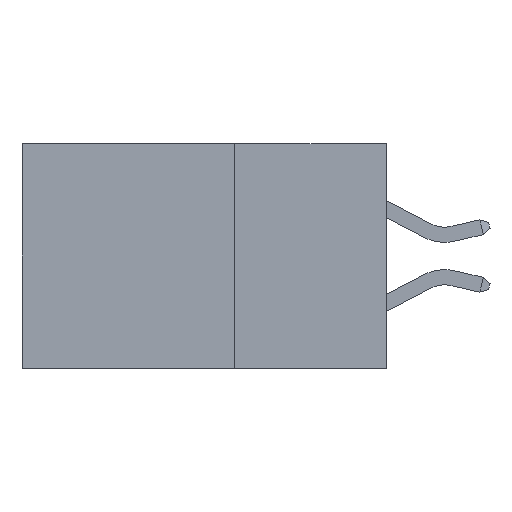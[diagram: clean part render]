
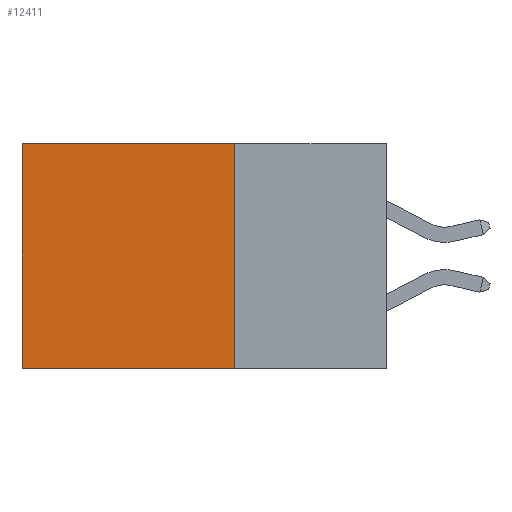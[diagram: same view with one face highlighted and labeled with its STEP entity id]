
A CAD part, left-side view. The second image highlights one B-rep face of the part: STEP entity #12411.
In plain terms, the highlighted planar face has unit normal (-1, 0, 0).
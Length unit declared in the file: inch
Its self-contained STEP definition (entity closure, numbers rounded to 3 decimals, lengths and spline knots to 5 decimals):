
#484 = CARTESIAN_POINT ( 'NONE',  ( 0.298, 0.6, 0. ) ) ;
#1757 = FACE_OUTER_BOUND ( 'NONE', #4726, .T. ) ;
#2132 = VERTEX_POINT ( 'NONE', #3837 ) ;
#2799 = VECTOR ( 'NONE', #9024, 39.37008 ) ;
#3102 = CARTESIAN_POINT ( 'NONE',  ( 0.298, 0.6, -0.37 ) ) ;
#3278 = ORIENTED_EDGE ( 'NONE', *, *, #11092, .F. ) ;
#3798 = VERTEX_POINT ( 'NONE', #9820 ) ;
#3837 = CARTESIAN_POINT ( 'NONE',  ( 0.298, 0.25, -0.37 ) ) ;
#4545 = VECTOR ( 'NONE', #10552, 39.37008 ) ;
#4726 = EDGE_LOOP ( 'NONE', ( #4836, #15436, #3278, #12036 ) ) ;
#4745 = LINE ( 'NONE', #8273, #10915 ) ;
#4836 = ORIENTED_EDGE ( 'NONE', *, *, #10391, .T. ) ;
#5254 = VECTOR ( 'NONE', #7885, 39.37008 ) ;
#5582 = EDGE_CURVE ( 'NONE', #2132, #15461, #14463, .T. ) ;
#5627 = CARTESIAN_POINT ( 'NONE',  ( 0.298, 0.25, 0. ) ) ;
#7170 = DIRECTION ( 'NONE',  ( 0., 1., 0. ) ) ;
#7885 = DIRECTION ( 'NONE',  ( 0., 1., 0. ) ) ;
#7887 = DIRECTION ( 'NONE',  ( 0., 0., -1. ) ) ;
#8273 = CARTESIAN_POINT ( 'NONE',  ( 0.298, 0.25, 0. ) ) ;
#9024 = DIRECTION ( 'NONE',  ( 0., 0., -1. ) ) ;
#9351 = CARTESIAN_POINT ( 'NONE',  ( 0.298, 0.6, 0. ) ) ;
#9820 = CARTESIAN_POINT ( 'NONE',  ( 0.298, 0.25, 0. ) ) ;
#10391 = EDGE_CURVE ( 'NONE', #11097, #15461, #10934, .T. ) ;
#10552 = DIRECTION ( 'NONE',  ( 0., 0., -1. ) ) ;
#10652 = AXIS2_PLACEMENT_3D ( 'NONE', #13872, #15311, #7887 ) ;
#10724 = EDGE_CURVE ( 'NONE', #3798, #11097, #4745, .T. ) ;
#10915 = VECTOR ( 'NONE', #7170, 39.37008 ) ;
#10934 = LINE ( 'NONE', #484, #2799 ) ;
#11092 = EDGE_CURVE ( 'NONE', #3798, #2132, #12046, .T. ) ;
#11097 = VERTEX_POINT ( 'NONE', #9351 ) ;
#12036 = ORIENTED_EDGE ( 'NONE', *, *, #10724, .T. ) ;
#12046 = LINE ( 'NONE', #5627, #4545 ) ;
#12411 = ADVANCED_FACE ( 'NONE', ( #1757 ), #12980, .F. ) ;
#12620 = CARTESIAN_POINT ( 'NONE',  ( 0.298, 0.25, -0.37 ) ) ;
#12980 = PLANE ( 'NONE',  #10652 ) ;
#13872 = CARTESIAN_POINT ( 'NONE',  ( 0.298, 0.25, 0. ) ) ;
#14463 = LINE ( 'NONE', #12620, #5254 ) ;
#15311 = DIRECTION ( 'NONE',  ( 1., 0., 0. ) ) ;
#15436 = ORIENTED_EDGE ( 'NONE', *, *, #5582, .F. ) ;
#15461 = VERTEX_POINT ( 'NONE', #3102 ) ;
